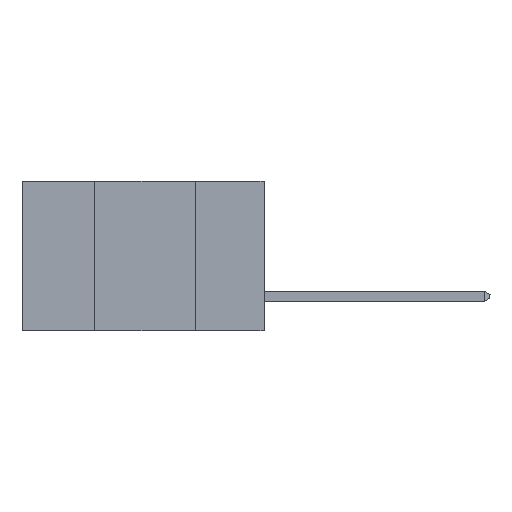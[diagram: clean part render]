
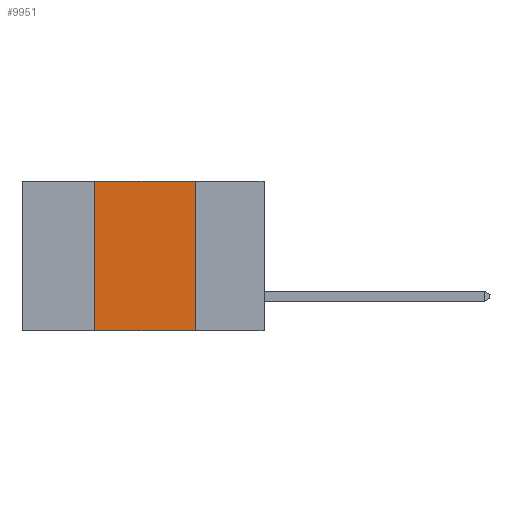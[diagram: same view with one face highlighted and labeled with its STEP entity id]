
A CAD part, left-side view. The second image highlights one B-rep face of the part: STEP entity #9951.
In plain terms, the highlighted planar face has unit normal (-1, 0, 0).
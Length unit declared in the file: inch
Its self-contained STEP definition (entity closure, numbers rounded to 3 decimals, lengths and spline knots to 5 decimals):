
#228 = CARTESIAN_POINT ( 'NONE',  ( 0., 0.42, 0. ) ) ;
#349 = VERTEX_POINT ( 'NONE', #10190 ) ;
#893 = EDGE_CURVE ( 'NONE', #1776, #349, #1061, .T. ) ;
#1061 = LINE ( 'NONE', #6009, #8592 ) ;
#1140 = FACE_OUTER_BOUND ( 'NONE', #1142, .T. ) ;
#1142 = EDGE_LOOP ( 'NONE', ( #1734, #6183, #8179, #1846 ) ) ;
#1182 = DIRECTION ( 'NONE',  ( 0., 0., 1. ) ) ;
#1572 = CARTESIAN_POINT ( 'NONE',  ( 0., 0.42, -0.37 ) ) ;
#1734 = ORIENTED_EDGE ( 'NONE', *, *, #2972, .F. ) ;
#1776 = VERTEX_POINT ( 'NONE', #1572 ) ;
#1846 = ORIENTED_EDGE ( 'NONE', *, *, #893, .T. ) ;
#2972 = EDGE_CURVE ( 'NONE', #9919, #349, #10996, .T. ) ;
#3036 = DIRECTION ( 'NONE',  ( 0., 0., -1. ) ) ;
#3160 = CARTESIAN_POINT ( 'NONE',  ( 0., 0.17, -0.37 ) ) ;
#3865 = LINE ( 'NONE', #6013, #8471 ) ;
#4591 = VERTEX_POINT ( 'NONE', #228 ) ;
#5186 = VECTOR ( 'NONE', #3036, 39.37008 ) ;
#5222 = CARTESIAN_POINT ( 'NONE',  ( 0., 0.17, 0. ) ) ;
#5731 = EDGE_CURVE ( 'NONE', #4591, #9919, #9209, .T. ) ;
#5973 = DIRECTION ( 'NONE',  ( 0., 0., -1. ) ) ;
#6009 = CARTESIAN_POINT ( 'NONE',  ( 0., 0.6, -0.37 ) ) ;
#6013 = CARTESIAN_POINT ( 'NONE',  ( 0., 0.42, -0.37 ) ) ;
#6094 = EDGE_CURVE ( 'NONE', #1776, #4591, #3865, .T. ) ;
#6162 = DIRECTION ( 'NONE',  ( 1., 0., 0. ) ) ;
#6183 = ORIENTED_EDGE ( 'NONE', *, *, #5731, .F. ) ;
#6837 = DIRECTION ( 'NONE',  ( 0., -1., 0. ) ) ;
#7090 = AXIS2_PLACEMENT_3D ( 'NONE', #10812, #6162, #5973 ) ;
#8179 = ORIENTED_EDGE ( 'NONE', *, *, #6094, .F. ) ;
#8257 = VECTOR ( 'NONE', #9147, 39.37008 ) ;
#8471 = VECTOR ( 'NONE', #1182, 39.37008 ) ;
#8592 = VECTOR ( 'NONE', #6837, 39.37008 ) ;
#9082 = PLANE ( 'NONE',  #7090 ) ;
#9147 = DIRECTION ( 'NONE',  ( 0., -1., 0. ) ) ;
#9209 = LINE ( 'NONE', #10995, #8257 ) ;
#9919 = VERTEX_POINT ( 'NONE', #5222 ) ;
#9951 = ADVANCED_FACE ( 'NONE', ( #1140 ), #9082, .F. ) ;
#10190 = CARTESIAN_POINT ( 'NONE',  ( 0., 0.17, -0.37 ) ) ;
#10812 = CARTESIAN_POINT ( 'NONE',  ( 0., 0.6, 0. ) ) ;
#10995 = CARTESIAN_POINT ( 'NONE',  ( 0., 0.6, 0. ) ) ;
#10996 = LINE ( 'NONE', #3160, #5186 ) ;
